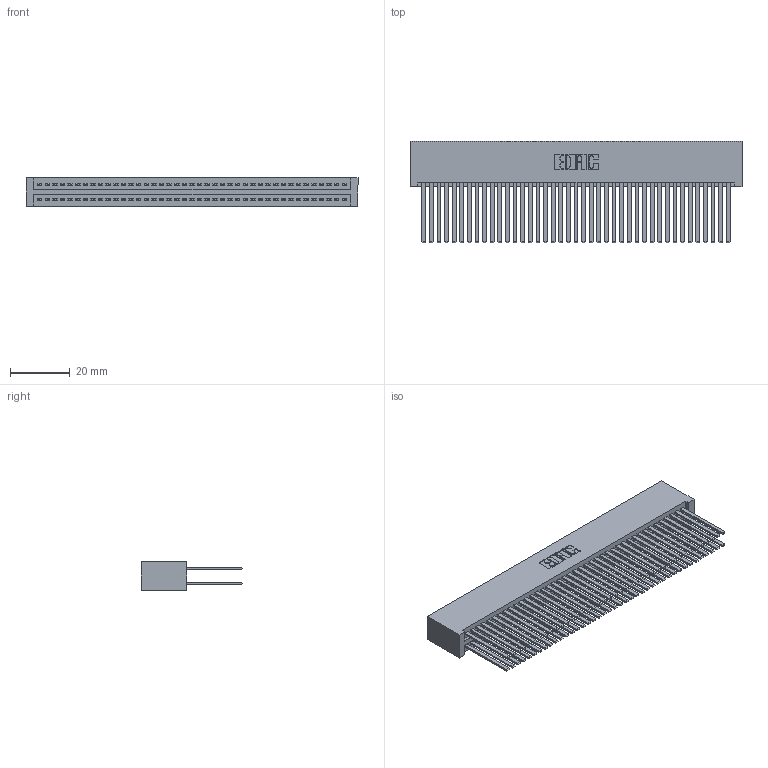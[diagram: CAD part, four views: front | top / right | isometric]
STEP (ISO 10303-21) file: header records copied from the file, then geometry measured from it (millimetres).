
FILE_DESCRIPTION (( 'STEP AP203' ), '1' );
FILE_NAME ('395-082-544-201.STEP', '2019-10-25T06:55:33', ( '' ), ( '' ), 'SwSTEP 2.0', 'SolidWorks 2016', '' );
FILE_SCHEMA (( 'CONFIG_CONTROL_DESIGN' ));
Length unit declared in the file: inch
Products named in the file (3): 345 Part_No Mounting Lugs; 345-292-001_345-293-144; 395-082-544-201
Assembly tree (83 placements, depth 2):
  395-082-544-201
    345 Part_No Mounting Lugs
    345-292-001_345-293-144  x82
Bounding box: 110.74 x 33.96 x 9.4 mm (x, y, z)
Volume: 12513.9 mm3; surface area: 22150.6 mm2
Topology: 83 solids, 83 shells, 3726 faces, 11059 edges, 7262 vertices
Faces by surface type: plane 2454, cylinder 1272
Entity records: 31843 total; most frequent: CARTESIAN_POINT 5336, ORIENTED_EDGE 5270, DIRECTION 4699, EDGE_CURVE 2635, VECTOR 2351, LINE 2351, VERTEX_POINT 1754, AXIS2_PLACEMENT_3D 1174
